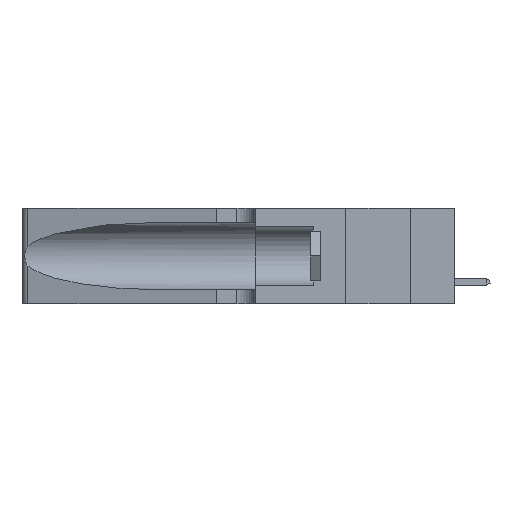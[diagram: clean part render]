
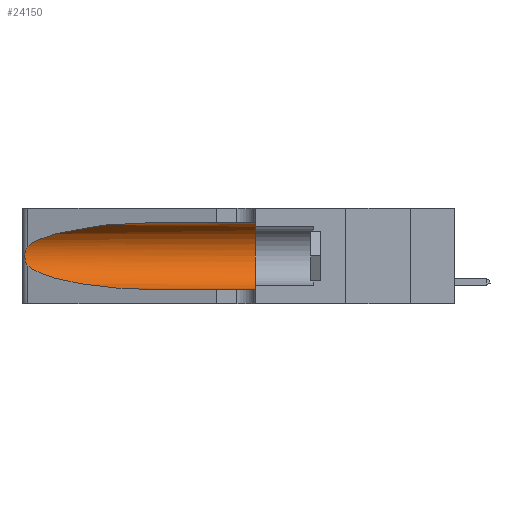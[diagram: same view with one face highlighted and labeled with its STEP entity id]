
A CAD part, left-side view. The second image highlights one B-rep face of the part: STEP entity #24150.
In plain terms, the highlighted cylindrical face has radius 3.308 mm (diameter 6.617 mm), a partial arc.
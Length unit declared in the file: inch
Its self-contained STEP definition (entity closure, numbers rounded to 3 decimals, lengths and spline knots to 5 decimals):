
#313 = CARTESIAN_POINT ( 'NONE',  ( 0.25639, 1.23184, 0.21858 ) ) ;
#1422 =( BOUNDED_CURVE ( )  B_SPLINE_CURVE ( 3, ( #30306, #6814, #46728, #42384 ),
 .UNSPECIFIED., .F., .F. ) 
 B_SPLINE_CURVE_WITH_KNOTS ( ( 4, 4 ),
 ( 1.5708, 2.84003 ),
 .UNSPECIFIED. ) 
 CURVE ( )  GEOMETRIC_REPRESENTATION_ITEM ( )  RATIONAL_B_SPLINE_CURVE ( ( 1., 0.87, 0.87, 1. ) ) 
 REPRESENTATION_ITEM ( '' )  );
#2304 = CYLINDRICAL_SURFACE ( 'NONE', #32550, 0.13025 ) ;
#2386 = CARTESIAN_POINT ( 'NONE',  ( 0.18966, 0.96281, 0.05475 ) ) ;
#2584 = LINE ( 'NONE', #9928, #6334 ) ;
#2592 = AXIS2_PLACEMENT_3D ( 'NONE', #25554, #37476, #26295 ) ;
#4340 = CARTESIAN_POINT ( 'NONE',  ( 0.25854, 1.2359, 0.20912 ) ) ;
#4494 = VERTEX_POINT ( 'NONE', #23988 ) ;
#4505 = EDGE_CURVE ( 'NONE', #16219, #26461, #9142, .T. ) ;
#5710 = CARTESIAN_POINT ( 'NONE',  ( 0.1305, 0.35, 0.05475 ) ) ;
#6334 = VECTOR ( 'NONE', #49629, 39.37008 ) ;
#6814 = CARTESIAN_POINT ( 'NONE',  ( 0.18966, 0.96281, 0.31525 ) ) ;
#7508 = CARTESIAN_POINT ( 'NONE',  ( 0.25789, 1.23486, 0.15765 ) ) ;
#9142 = B_SPLINE_CURVE_WITH_KNOTS ( 'NONE', 3,
 ( #15785, #43778, #313, #28319, #4340, #19934, #16100, #44084, #32189, #19613, #7508, #39601, #40077, #23826 ),
 .UNSPECIFIED., .F., .F.,
 ( 4, 2, 2, 2, 2, 2, 4 ),
 ( 0., 0.00027, 0.00053, 0.00107, 0.0016, 0.00187, 0.00214 ),
 .UNSPECIFIED. ) ;
#9928 = CARTESIAN_POINT ( 'NONE',  ( 0.1305, 1.61858, 0.31525 ) ) ;
#10624 = CARTESIAN_POINT ( 'NONE',  ( 0.25487, 1.22718, 0.14631 ) ) ;
#10914 = ORIENTED_EDGE ( 'NONE', *, *, #18015, .T. ) ;
#11998 = CARTESIAN_POINT ( 'NONE',  ( 0.1305, 0.35, 0.31525 ) ) ;
#12715 = ORIENTED_EDGE ( 'NONE', *, *, #21822, .T. ) ;
#14716 = DIRECTION ( 'NONE',  ( 0., -1., 0. ) ) ;
#14906 = CARTESIAN_POINT ( 'NONE',  ( 0.1305, 1.61858, 0.185 ) ) ;
#15785 = CARTESIAN_POINT ( 'NONE',  ( 0.25487, 1.22718, 0.22369 ) ) ;
#16100 = CARTESIAN_POINT ( 'NONE',  ( 0.26075, 1.23896, 0.19203 ) ) ;
#16219 = VERTEX_POINT ( 'NONE', #41629 ) ;
#18015 = EDGE_CURVE ( 'NONE', #34202, #41838, #49263, .T. ) ;
#18187 = CARTESIAN_POINT ( 'NONE',  ( 0.1305, 0.72297, 0.05475 ) ) ;
#19529 = EDGE_CURVE ( 'NONE', #41014, #41838, #46058, .T. ) ;
#19613 = CARTESIAN_POINT ( 'NONE',  ( 0.25856, 1.23593, 0.16098 ) ) ;
#19934 = CARTESIAN_POINT ( 'NONE',  ( 0.26018, 1.23835, 0.19895 ) ) ;
#21403 = EDGE_CURVE ( 'NONE', #4494, #41014, #2584, .T. ) ;
#21822 = EDGE_CURVE ( 'NONE', #4494, #16219, #1422, .T. ) ;
#22696 = CARTESIAN_POINT ( 'NONE',  ( 0.2373, 1.15595, 0.08982 ) ) ;
#23826 = CARTESIAN_POINT ( 'NONE',  ( 0.25487, 1.22718, 0.14631 ) ) ;
#23988 = CARTESIAN_POINT ( 'NONE',  ( 0.1305, 0.72297, 0.31525 ) ) ;
#24150 = ADVANCED_FACE ( 'NONE', ( #51798 ), #2304, .F. ) ;
#25554 = CARTESIAN_POINT ( 'NONE',  ( 0.1305, 0.35, 0.185 ) ) ;
#26295 = DIRECTION ( 'NONE',  ( 0., 0., 1. ) ) ;
#26461 = VERTEX_POINT ( 'NONE', #47058 ) ;
#28019 = VECTOR ( 'NONE', #43473, 39.37008 ) ;
#28153 = ORIENTED_EDGE ( 'NONE', *, *, #19529, .F. ) ;
#28319 = CARTESIAN_POINT ( 'NONE',  ( 0.25787, 1.23484, 0.2124 ) ) ;
#28952 = ORIENTED_EDGE ( 'NONE', *, *, #4505, .T. ) ;
#30306 = CARTESIAN_POINT ( 'NONE',  ( 0.1305, 0.72297, 0.31525 ) ) ;
#30907 = CARTESIAN_POINT ( 'NONE',  ( 0.1305, 0.72297, 0.05475 ) ) ;
#31379 = EDGE_LOOP ( 'NONE', ( #12715, #28952, #40942, #10914, #28153, #43478 ) ) ;
#32139 = CARTESIAN_POINT ( 'NONE',  ( 0.1305, 1.61858, 0.05475 ) ) ;
#32189 = CARTESIAN_POINT ( 'NONE',  ( 0.26017, 1.23833, 0.17102 ) ) ;
#32550 = AXIS2_PLACEMENT_3D ( 'NONE', #14906, #14716, #42686 ) ;
#34202 = VERTEX_POINT ( 'NONE', #18187 ) ;
#37476 = DIRECTION ( 'NONE',  ( 0., 1., 0. ) ) ;
#39601 = CARTESIAN_POINT ( 'NONE',  ( 0.25639, 1.23186, 0.15144 ) ) ;
#39918 = EDGE_CURVE ( 'NONE', #26461, #34202, #47366, .T. ) ;
#40077 = CARTESIAN_POINT ( 'NONE',  ( 0.25555, 1.22993, 0.14849 ) ) ;
#40942 = ORIENTED_EDGE ( 'NONE', *, *, #39918, .T. ) ;
#41014 = VERTEX_POINT ( 'NONE', #11998 ) ;
#41629 = CARTESIAN_POINT ( 'NONE',  ( 0.25487, 1.22718, 0.22369 ) ) ;
#41838 = VERTEX_POINT ( 'NONE', #5710 ) ;
#42384 = CARTESIAN_POINT ( 'NONE',  ( 0.25487, 1.22718, 0.22369 ) ) ;
#42686 = DIRECTION ( 'NONE',  ( 0., 0., -1. ) ) ;
#43473 = DIRECTION ( 'NONE',  ( 0., -1., 0. ) ) ;
#43478 = ORIENTED_EDGE ( 'NONE', *, *, #21403, .F. ) ;
#43778 = CARTESIAN_POINT ( 'NONE',  ( 0.25555, 1.22994, 0.2215 ) ) ;
#44084 = CARTESIAN_POINT ( 'NONE',  ( 0.26075, 1.23896, 0.178 ) ) ;
#46058 = CIRCLE ( 'NONE', #2592, 0.13025 ) ;
#46728 = CARTESIAN_POINT ( 'NONE',  ( 0.2373, 1.15595, 0.28018 ) ) ;
#47058 = CARTESIAN_POINT ( 'NONE',  ( 0.25487, 1.22718, 0.14631 ) ) ;
#47366 =( BOUNDED_CURVE ( )  B_SPLINE_CURVE ( 3, ( #10624, #22696, #2386, #30907 ),
 .UNSPECIFIED., .F., .F. ) 
 B_SPLINE_CURVE_WITH_KNOTS ( ( 4, 4 ),
 ( 3.44316, 4.71239 ),
 .UNSPECIFIED. ) 
 CURVE ( )  GEOMETRIC_REPRESENTATION_ITEM ( )  RATIONAL_B_SPLINE_CURVE ( ( 1., 0.87, 0.87, 1. ) ) 
 REPRESENTATION_ITEM ( '' )  );
#49263 = LINE ( 'NONE', #32139, #28019 ) ;
#49629 = DIRECTION ( 'NONE',  ( 0., -1., 0. ) ) ;
#51798 = FACE_OUTER_BOUND ( 'NONE', #31379, .T. ) ;
